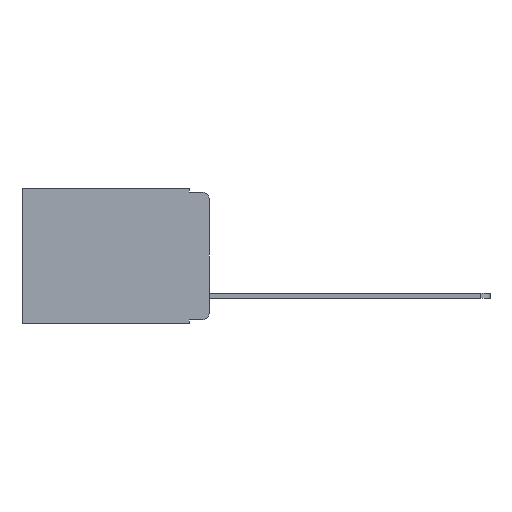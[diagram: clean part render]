
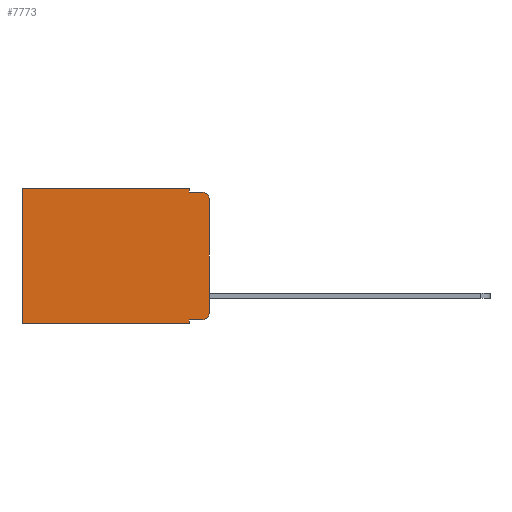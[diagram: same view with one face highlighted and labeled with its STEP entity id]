
A CAD part, left-side view. The second image highlights one B-rep face of the part: STEP entity #7773.
In plain terms, the highlighted planar face has unit normal (-1, 0, 0).
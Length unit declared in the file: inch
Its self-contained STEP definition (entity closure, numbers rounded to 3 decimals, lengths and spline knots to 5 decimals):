
#3 = ORIENTED_EDGE ( 'NONE', *, *, #8201, .T. ) ;
#275 = VERTEX_POINT ( 'NONE', #9870 ) ;
#298 = VECTOR ( 'NONE', #6468, 39.37008 ) ;
#359 = CARTESIAN_POINT ( 'NONE',  ( 0.298, 0., -0.343 ) ) ;
#455 = LINE ( 'NONE', #9492, #9605 ) ;
#620 = ORIENTED_EDGE ( 'NONE', *, *, #2396, .F. ) ;
#766 = DIRECTION ( 'NONE',  ( 0., 0., -1. ) ) ;
#824 = ORIENTED_EDGE ( 'NONE', *, *, #9614, .F. ) ;
#842 = CARTESIAN_POINT ( 'NONE',  ( 0.298, 0., 0. ) ) ;
#926 = CARTESIAN_POINT ( 'NONE',  ( 0.298, 0., 0. ) ) ;
#1009 = DIRECTION ( 'NONE',  ( 0., 0., -1. ) ) ;
#1043 = CARTESIAN_POINT ( 'NONE',  ( 0.298, 0.02, -0.333 ) ) ;
#1202 = DIRECTION ( 'NONE',  ( 0., -1., 0. ) ) ;
#1206 = VERTEX_POINT ( 'NONE', #1316 ) ;
#1227 = EDGE_CURVE ( 'NONE', #9699, #5008, #8994, .T. ) ;
#1238 = AXIS2_PLACEMENT_3D ( 'NONE', #926, #3719, #9707 ) ;
#1289 = CARTESIAN_POINT ( 'NONE',  ( 0.298, 0.051, -0.333 ) ) ;
#1316 = CARTESIAN_POINT ( 'NONE',  ( 0.298, 0., -0.313 ) ) ;
#1332 = ORIENTED_EDGE ( 'NONE', *, *, #5503, .F. ) ;
#1683 = DIRECTION ( 'NONE',  ( 0., 1., 0. ) ) ;
#1796 = VERTEX_POINT ( 'NONE', #1043 ) ;
#2167 = LINE ( 'NONE', #9374, #10958 ) ;
#2280 = VERTEX_POINT ( 'NONE', #8513 ) ;
#2396 = EDGE_CURVE ( 'NONE', #4172, #9699, #10842, .T. ) ;
#2532 = EDGE_CURVE ( 'NONE', #2280, #275, #7675, .T. ) ;
#2620 = EDGE_CURVE ( 'NONE', #4172, #2280, #2167, .T. ) ;
#2671 = DIRECTION ( 'NONE',  ( -1., 0., 0. ) ) ;
#2682 = DIRECTION ( 'NONE',  ( -1., 0., 0. ) ) ;
#2685 = CARTESIAN_POINT ( 'NONE',  ( 0.298, 0.02, -0.03 ) ) ;
#2879 = FACE_OUTER_BOUND ( 'NONE', #4937, .T. ) ;
#3241 = VECTOR ( 'NONE', #9266, 39.37008 ) ;
#3340 = CARTESIAN_POINT ( 'NONE',  ( 0.298, 0.051, -0.01 ) ) ;
#3552 = LINE ( 'NONE', #359, #3241 ) ;
#3588 = CARTESIAN_POINT ( 'NONE',  ( 0.298, 0.473, 0. ) ) ;
#3631 = ORIENTED_EDGE ( 'NONE', *, *, #4331, .T. ) ;
#3719 = DIRECTION ( 'NONE',  ( 1., 0., 0. ) ) ;
#3756 = EDGE_CURVE ( 'NONE', #9052, #5008, #4116, .T. ) ;
#4065 = CARTESIAN_POINT ( 'NONE',  ( 0.298, 0., -0.03 ) ) ;
#4116 = CIRCLE ( 'NONE', #5112, 0.02 ) ;
#4172 = VERTEX_POINT ( 'NONE', #10529 ) ;
#4191 = DIRECTION ( 'NONE',  ( 0., 0., -1. ) ) ;
#4226 = CARTESIAN_POINT ( 'NONE',  ( 0.298, 0.051, -0.01 ) ) ;
#4331 = EDGE_CURVE ( 'NONE', #11058, #1796, #455, .T. ) ;
#4619 = VECTOR ( 'NONE', #766, 39.37008 ) ;
#4937 = EDGE_LOOP ( 'NONE', ( #1332, #8628, #5336, #620, #8492, #5085, #824, #8740, #3631, #3 ) ) ;
#5008 = VERTEX_POINT ( 'NONE', #9141 ) ;
#5085 = ORIENTED_EDGE ( 'NONE', *, *, #2532, .T. ) ;
#5112 = AXIS2_PLACEMENT_3D ( 'NONE', #2685, #2682, #5790 ) ;
#5186 = LINE ( 'NONE', #8992, #298 ) ;
#5336 = ORIENTED_EDGE ( 'NONE', *, *, #1227, .F. ) ;
#5353 = VECTOR ( 'NONE', #4191, 39.37008 ) ;
#5503 = EDGE_CURVE ( 'NONE', #9052, #1206, #6699, .T. ) ;
#5617 = AXIS2_PLACEMENT_3D ( 'NONE', #7917, #2671, #8780 ) ;
#5790 = DIRECTION ( 'NONE',  ( 0., 0., -1. ) ) ;
#6468 = DIRECTION ( 'NONE',  ( 0., 0., -1. ) ) ;
#6600 = CARTESIAN_POINT ( 'NONE',  ( 0.298, 0.051, 0. ) ) ;
#6699 = LINE ( 'NONE', #842, #4619 ) ;
#7672 = VERTEX_POINT ( 'NONE', #8722 ) ;
#7675 = LINE ( 'NONE', #3588, #5353 ) ;
#7773 = ADVANCED_FACE ( 'NONE', ( #2879 ), #11220, .F. ) ;
#7917 = CARTESIAN_POINT ( 'NONE',  ( 0.298, 0.02, -0.313 ) ) ;
#8201 = EDGE_CURVE ( 'NONE', #1796, #1206, #9360, .T. ) ;
#8368 = EDGE_CURVE ( 'NONE', #11058, #7672, #5186, .T. ) ;
#8492 = ORIENTED_EDGE ( 'NONE', *, *, #2620, .T. ) ;
#8513 = CARTESIAN_POINT ( 'NONE',  ( 0.298, 0.473, 0. ) ) ;
#8628 = ORIENTED_EDGE ( 'NONE', *, *, #3756, .T. ) ;
#8722 = CARTESIAN_POINT ( 'NONE',  ( 0.298, 0.051, -0.343 ) ) ;
#8739 = VECTOR ( 'NONE', #1202, 39.37008 ) ;
#8740 = ORIENTED_EDGE ( 'NONE', *, *, #8368, .F. ) ;
#8755 = VECTOR ( 'NONE', #1009, 39.37008 ) ;
#8780 = DIRECTION ( 'NONE',  ( 0., 0., -1. ) ) ;
#8992 = CARTESIAN_POINT ( 'NONE',  ( 0.298, 0.051, 0. ) ) ;
#8994 = LINE ( 'NONE', #4226, #8739 ) ;
#9052 = VERTEX_POINT ( 'NONE', #4065 ) ;
#9141 = CARTESIAN_POINT ( 'NONE',  ( 0.298, 0.02, -0.01 ) ) ;
#9266 = DIRECTION ( 'NONE',  ( 0., 1., 0. ) ) ;
#9360 = CIRCLE ( 'NONE', #5617, 0.02 ) ;
#9374 = CARTESIAN_POINT ( 'NONE',  ( 0.298, 0., 0. ) ) ;
#9492 = CARTESIAN_POINT ( 'NONE',  ( 0.298, 0.051, -0.333 ) ) ;
#9496 = DIRECTION ( 'NONE',  ( 0., -1., 0. ) ) ;
#9605 = VECTOR ( 'NONE', #9496, 39.37008 ) ;
#9614 = EDGE_CURVE ( 'NONE', #7672, #275, #3552, .T. ) ;
#9699 = VERTEX_POINT ( 'NONE', #3340 ) ;
#9707 = DIRECTION ( 'NONE',  ( 0., 0., -1. ) ) ;
#9870 = CARTESIAN_POINT ( 'NONE',  ( 0.298, 0.473, -0.343 ) ) ;
#10529 = CARTESIAN_POINT ( 'NONE',  ( 0.298, 0.051, 0. ) ) ;
#10842 = LINE ( 'NONE', #6600, #8755 ) ;
#10958 = VECTOR ( 'NONE', #1683, 39.37008 ) ;
#11058 = VERTEX_POINT ( 'NONE', #1289 ) ;
#11220 = PLANE ( 'NONE',  #1238 ) ;
